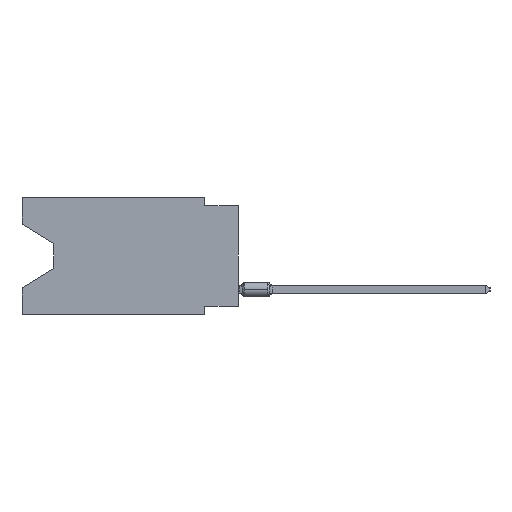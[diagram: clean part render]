
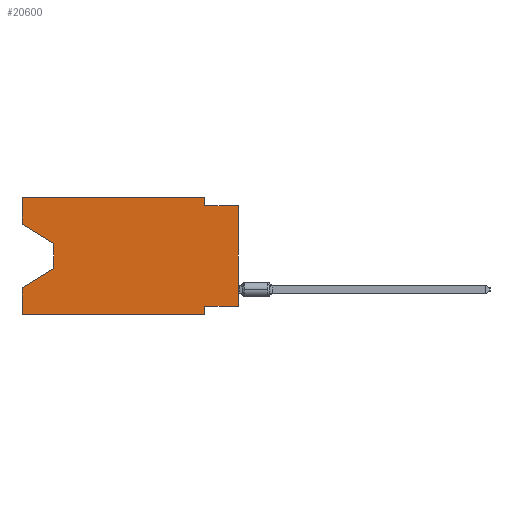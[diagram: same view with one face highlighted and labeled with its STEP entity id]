
A CAD part, left-side view. The second image highlights one B-rep face of the part: STEP entity #20600.
In plain terms, the highlighted planar face has unit normal (-1, 0, 0).
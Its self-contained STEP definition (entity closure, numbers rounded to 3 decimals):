
#390 = VECTOR ( 'NONE', #24565, 1000. ) ;
#797 = CARTESIAN_POINT ( 'NONE',  ( 0., 2.54, -0.635 ) ) ;
#915 = CARTESIAN_POINT ( 'NONE',  ( 0., 16.383, 0. ) ) ;
#974 = DIRECTION ( 'NONE',  ( 1., 0., 0. ) ) ;
#1071 = LINE ( 'NONE', #29848, #7955 ) ;
#1332 = DIRECTION ( 'NONE',  ( 0., 0., -1. ) ) ;
#1900 = DIRECTION ( 'NONE',  ( 0., 0., 1. ) ) ;
#2150 = CARTESIAN_POINT ( 'NONE',  ( 0., 16.383, -2.038 ) ) ;
#2151 = VERTEX_POINT ( 'NONE', #29057 ) ;
#2642 = LINE ( 'NONE', #33633, #10503 ) ;
#2858 = ORIENTED_EDGE ( 'NONE', *, *, #18265, .T. ) ;
#2959 = DIRECTION ( 'NONE',  ( 0., 0., -1. ) ) ;
#3660 = CARTESIAN_POINT ( 'NONE',  ( 0., 0., -8.255 ) ) ;
#3962 = VERTEX_POINT ( 'NONE', #30891 ) ;
#4141 = CARTESIAN_POINT ( 'NONE',  ( 0., 0., 0. ) ) ;
#4706 = PLANE ( 'NONE',  #28730 ) ;
#5208 = VECTOR ( 'NONE', #21912, 1000. ) ;
#5218 = VECTOR ( 'NONE', #2959, 1000. ) ;
#5541 = VERTEX_POINT ( 'NONE', #16390 ) ;
#5559 = CARTESIAN_POINT ( 'NONE',  ( 0., 16.383, 0. ) ) ;
#5805 = ORIENTED_EDGE ( 'NONE', *, *, #26730, .T. ) ;
#6303 = EDGE_CURVE ( 'NONE', #13495, #11517, #1071, .T. ) ;
#6516 = CARTESIAN_POINT ( 'NONE',  ( 0., 0., -0.635 ) ) ;
#6581 = VERTEX_POINT ( 'NONE', #21166 ) ;
#6629 = LINE ( 'NONE', #3660, #30941 ) ;
#6847 = CARTESIAN_POINT ( 'NONE',  ( 0., 2.54, 0. ) ) ;
#6884 = VERTEX_POINT ( 'NONE', #34674 ) ;
#7333 = ORIENTED_EDGE ( 'NONE', *, *, #16546, .T. ) ;
#7408 = EDGE_CURVE ( 'NONE', #11517, #10775, #35000, .T. ) ;
#7955 = VECTOR ( 'NONE', #32255, 1000. ) ;
#8790 = VERTEX_POINT ( 'NONE', #915 ) ;
#8856 = VECTOR ( 'NONE', #1332, 1000. ) ;
#9100 = CARTESIAN_POINT ( 'NONE',  ( 0., 16.383, -8.89 ) ) ;
#9763 = DIRECTION ( 'NONE',  ( 0., 1., 0. ) ) ;
#9767 = VECTOR ( 'NONE', #15710, 1000. ) ;
#9925 = LINE ( 'NONE', #21263, #15302 ) ;
#10248 = EDGE_CURVE ( 'NONE', #6884, #2151, #12853, .T. ) ;
#10503 = VECTOR ( 'NONE', #22318, 1000. ) ;
#10775 = VERTEX_POINT ( 'NONE', #18897 ) ;
#11517 = VERTEX_POINT ( 'NONE', #18019 ) ;
#12853 = LINE ( 'NONE', #15272, #8856 ) ;
#13246 = LINE ( 'NONE', #24196, #390 ) ;
#13495 = VERTEX_POINT ( 'NONE', #2150 ) ;
#13752 = ORIENTED_EDGE ( 'NONE', *, *, #28189, .F. ) ;
#14578 = ORIENTED_EDGE ( 'NONE', *, *, #36529, .F. ) ;
#14714 = ORIENTED_EDGE ( 'NONE', *, *, #10248, .F. ) ;
#14807 = VECTOR ( 'NONE', #1900, 1000. ) ;
#15272 = CARTESIAN_POINT ( 'NONE',  ( 0., 2.54, -8.89 ) ) ;
#15302 = VECTOR ( 'NONE', #32587, 1000. ) ;
#15375 = EDGE_CURVE ( 'NONE', #3962, #6884, #6629, .T. ) ;
#15663 = FACE_OUTER_BOUND ( 'NONE', #35514, .T. ) ;
#15710 = DIRECTION ( 'NONE',  ( 0., 0., -1. ) ) ;
#15848 = DIRECTION ( 'NONE',  ( 0., 0., -1. ) ) ;
#16390 = CARTESIAN_POINT ( 'NONE',  ( 0., 0., -0.635 ) ) ;
#16546 = EDGE_CURVE ( 'NONE', #10775, #6581, #13246, .T. ) ;
#17315 = ORIENTED_EDGE ( 'NONE', *, *, #7408, .T. ) ;
#17707 = ORIENTED_EDGE ( 'NONE', *, *, #6303, .T. ) ;
#18019 = CARTESIAN_POINT ( 'NONE',  ( 0., 13.97, -3.505 ) ) ;
#18127 = CARTESIAN_POINT ( 'NONE',  ( 0., 13.97, -3.505 ) ) ;
#18233 = CARTESIAN_POINT ( 'NONE',  ( 0., 16.383, -8.89 ) ) ;
#18265 = EDGE_CURVE ( 'NONE', #28161, #2151, #29345, .T. ) ;
#18897 = CARTESIAN_POINT ( 'NONE',  ( 0., 13.97, -5.385 ) ) ;
#20266 = ORIENTED_EDGE ( 'NONE', *, *, #15375, .F. ) ;
#20600 = ADVANCED_FACE ( 'NONE', ( #15663 ), #4706, .F. ) ;
#21166 = CARTESIAN_POINT ( 'NONE',  ( 0., 16.383, -6.852 ) ) ;
#21263 = CARTESIAN_POINT ( 'NONE',  ( 0., 16.383, 0. ) ) ;
#21856 = CARTESIAN_POINT ( 'NONE',  ( 0., 2.54, 0. ) ) ;
#21912 = DIRECTION ( 'NONE',  ( 0., -1., 0. ) ) ;
#22318 = DIRECTION ( 'NONE',  ( 0., 0., 1. ) ) ;
#22337 = VERTEX_POINT ( 'NONE', #797 ) ;
#22625 = LINE ( 'NONE', #21856, #5218 ) ;
#22631 = EDGE_CURVE ( 'NONE', #28161, #6581, #2642, .T. ) ;
#23404 = DIRECTION ( 'NONE',  ( 0., -1., 0. ) ) ;
#23420 = DIRECTION ( 'NONE',  ( 0., -1., 0. ) ) ;
#24196 = CARTESIAN_POINT ( 'NONE',  ( 0., 13.97, -5.385 ) ) ;
#24353 = ORIENTED_EDGE ( 'NONE', *, *, #28482, .F. ) ;
#24535 = VERTEX_POINT ( 'NONE', #6847 ) ;
#24565 = DIRECTION ( 'NONE',  ( 0., 0.855, -0.519 ) ) ;
#26730 = EDGE_CURVE ( 'NONE', #3962, #5541, #30111, .T. ) ;
#26964 = CARTESIAN_POINT ( 'NONE',  ( 0., 16.383, 0. ) ) ;
#27093 = VECTOR ( 'NONE', #23404, 1000. ) ;
#28161 = VERTEX_POINT ( 'NONE', #9100 ) ;
#28189 = EDGE_CURVE ( 'NONE', #22337, #5541, #31746, .T. ) ;
#28482 = EDGE_CURVE ( 'NONE', #8790, #24535, #36184, .T. ) ;
#28730 = AXIS2_PLACEMENT_3D ( 'NONE', #26964, #974, #15848 ) ;
#29057 = CARTESIAN_POINT ( 'NONE',  ( 0., 2.54, -8.89 ) ) ;
#29176 = EDGE_CURVE ( 'NONE', #13495, #8790, #9925, .T. ) ;
#29204 = VECTOR ( 'NONE', #23420, 1000. ) ;
#29345 = LINE ( 'NONE', #18233, #29204 ) ;
#29848 = CARTESIAN_POINT ( 'NONE',  ( 0., 16.383, -2.038 ) ) ;
#30111 = LINE ( 'NONE', #4141, #14807 ) ;
#30891 = CARTESIAN_POINT ( 'NONE',  ( 0., 0., -8.255 ) ) ;
#30941 = VECTOR ( 'NONE', #9763, 1000. ) ;
#31746 = LINE ( 'NONE', #6516, #27093 ) ;
#32255 = DIRECTION ( 'NONE',  ( 0., -0.855, -0.519 ) ) ;
#32587 = DIRECTION ( 'NONE',  ( 0., 0., 1. ) ) ;
#32892 = ORIENTED_EDGE ( 'NONE', *, *, #22631, .F. ) ;
#33633 = CARTESIAN_POINT ( 'NONE',  ( 0., 16.383, 0. ) ) ;
#34674 = CARTESIAN_POINT ( 'NONE',  ( 0., 2.54, -8.255 ) ) ;
#34946 = ORIENTED_EDGE ( 'NONE', *, *, #29176, .F. ) ;
#35000 = LINE ( 'NONE', #18127, #9767 ) ;
#35514 = EDGE_LOOP ( 'NONE', ( #17707, #17315, #7333, #32892, #2858, #14714, #20266, #5805, #13752, #14578, #24353, #34946 ) ) ;
#36184 = LINE ( 'NONE', #5559, #5208 ) ;
#36529 = EDGE_CURVE ( 'NONE', #24535, #22337, #22625, .T. ) ;
